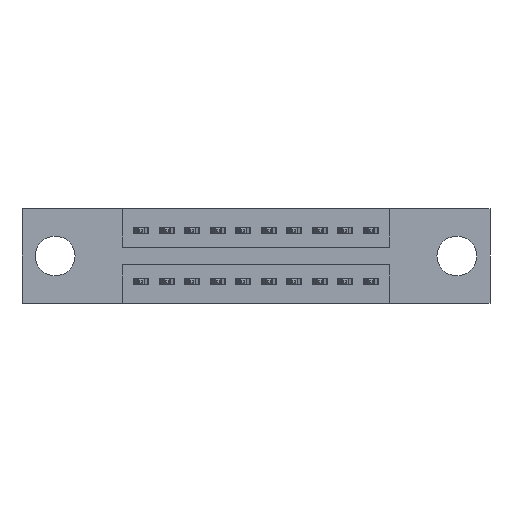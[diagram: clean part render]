
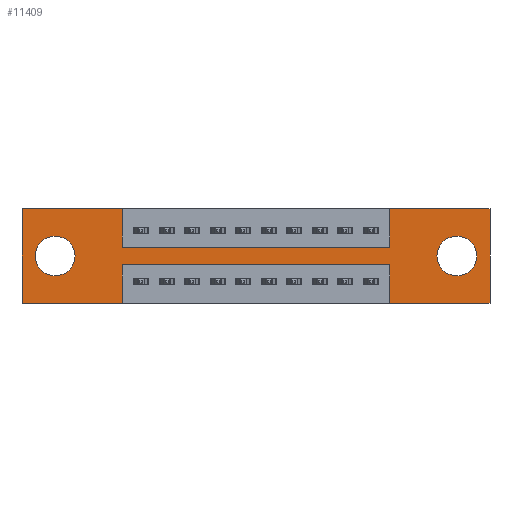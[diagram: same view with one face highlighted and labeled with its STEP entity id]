
A CAD part, front view. The second image highlights one B-rep face of the part: STEP entity #11409.
In plain terms, the highlighted planar face has unit normal (0, -1, 0).
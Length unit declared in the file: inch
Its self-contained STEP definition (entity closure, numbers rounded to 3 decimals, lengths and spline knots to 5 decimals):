
#39 = LINE ( 'NONE', #8794, #2908 ) ;
#45 = CARTESIAN_POINT ( 'NONE',  ( 0.3925, 0., -0.37 ) ) ;
#82 = CARTESIAN_POINT ( 'NONE',  ( 0., 0., 0. ) ) ;
#145 = CARTESIAN_POINT ( 'NONE',  ( 1.4425, 0., 0. ) ) ;
#156 = CARTESIAN_POINT ( 'NONE',  ( 0., 0., 0. ) ) ;
#295 = CIRCLE ( 'NONE', #908, 0.078 ) ;
#339 = DIRECTION ( 'NONE',  ( 1., 0., 0. ) ) ;
#346 = DIRECTION ( 'NONE',  ( 0., 0., 1. ) ) ;
#673 = VERTEX_POINT ( 'NONE', #9736 ) ;
#859 = ORIENTED_EDGE ( 'NONE', *, *, #5480, .T. ) ;
#908 = AXIS2_PLACEMENT_3D ( 'NONE', #1047, #8847, #7703 ) ;
#933 = LINE ( 'NONE', #156, #1925 ) ;
#968 = ORIENTED_EDGE ( 'NONE', *, *, #11265, .T. ) ;
#1047 = CARTESIAN_POINT ( 'NONE',  ( 1.705, 0., -0.185 ) ) ;
#1105 = LINE ( 'NONE', #9616, #3787 ) ;
#1170 = CARTESIAN_POINT ( 'NONE',  ( 0., 0., 0. ) ) ;
#1221 = DIRECTION ( 'NONE',  ( 0., 0., -1. ) ) ;
#1222 = ORIENTED_EDGE ( 'NONE', *, *, #12568, .T. ) ;
#1416 = VECTOR ( 'NONE', #346, 39.37008 ) ;
#1449 = LINE ( 'NONE', #5335, #8667 ) ;
#1576 = VERTEX_POINT ( 'NONE', #10463 ) ;
#1659 = PLANE ( 'NONE',  #2640 ) ;
#1796 = ORIENTED_EDGE ( 'NONE', *, *, #3796, .F. ) ;
#1900 = CARTESIAN_POINT ( 'NONE',  ( 1.4425, 0., -0.37 ) ) ;
#1903 = VERTEX_POINT ( 'NONE', #8295 ) ;
#1925 = VECTOR ( 'NONE', #5719, 39.37008 ) ;
#2301 = EDGE_CURVE ( 'NONE', #10775, #4617, #4600, .T. ) ;
#2331 = DIRECTION ( 'NONE',  ( 1., 0., 0. ) ) ;
#2640 = AXIS2_PLACEMENT_3D ( 'NONE', #3624, #9512, #3561 ) ;
#2673 = FACE_BOUND ( 'NONE', #9691, .T. ) ;
#2891 = DIRECTION ( 'NONE',  ( 0., 0., -1. ) ) ;
#2908 = VECTOR ( 'NONE', #8858, 39.37008 ) ;
#2923 = CARTESIAN_POINT ( 'NONE',  ( 0.13, 0., -0.263 ) ) ;
#3191 = EDGE_LOOP ( 'NONE', ( #4828, #6863, #5349, #1796, #12527, #7733, #8621, #10648, #10060, #8005, #12180, #5104 ) ) ;
#3241 = ORIENTED_EDGE ( 'NONE', *, *, #4675, .T. ) ;
#3254 = VERTEX_POINT ( 'NONE', #12557 ) ;
#3561 = DIRECTION ( 'NONE',  ( 0., 0., -1. ) ) ;
#3624 = CARTESIAN_POINT ( 'NONE',  ( 0., 0., -0.37 ) ) ;
#3642 = CARTESIAN_POINT ( 'NONE',  ( 0.3925, 0., -0.22 ) ) ;
#3662 = CIRCLE ( 'NONE', #6130, 0.078 ) ;
#3787 = VECTOR ( 'NONE', #11760, 39.37008 ) ;
#3796 = EDGE_CURVE ( 'NONE', #10252, #10162, #39, .T. ) ;
#3860 = CARTESIAN_POINT ( 'NONE',  ( 1.835, 0., -0.37 ) ) ;
#3870 = CARTESIAN_POINT ( 'NONE',  ( 0.3925, 0., -0.22 ) ) ;
#3967 = CARTESIAN_POINT ( 'NONE',  ( 1.835, 0., 0. ) ) ;
#4052 = DIRECTION ( 'NONE',  ( 0., 0., -1. ) ) ;
#4404 = EDGE_LOOP ( 'NONE', ( #1222, #3241 ) ) ;
#4547 = CIRCLE ( 'NONE', #5791, 0.078 ) ;
#4600 = LINE ( 'NONE', #3642, #11248 ) ;
#4617 = VERTEX_POINT ( 'NONE', #3870 ) ;
#4675 = EDGE_CURVE ( 'NONE', #9756, #10533, #4547, .T. ) ;
#4795 = EDGE_CURVE ( 'NONE', #10442, #5657, #1449, .T. ) ;
#4828 = ORIENTED_EDGE ( 'NONE', *, *, #8681, .F. ) ;
#5051 = LINE ( 'NONE', #145, #7648 ) ;
#5060 = EDGE_CURVE ( 'NONE', #1576, #10442, #933, .T. ) ;
#5104 = ORIENTED_EDGE ( 'NONE', *, *, #10304, .F. ) ;
#5241 = DIRECTION ( 'NONE',  ( 0., 0., 1. ) ) ;
#5259 = CARTESIAN_POINT ( 'NONE',  ( 0., 0., -0.37 ) ) ;
#5335 = CARTESIAN_POINT ( 'NONE',  ( 0., 0., 0. ) ) ;
#5349 = ORIENTED_EDGE ( 'NONE', *, *, #12106, .F. ) ;
#5400 = EDGE_CURVE ( 'NONE', #5657, #5859, #9602, .T. ) ;
#5480 = EDGE_CURVE ( 'NONE', #1903, #3254, #295, .T. ) ;
#5517 = VERTEX_POINT ( 'NONE', #3967 ) ;
#5569 = EDGE_CURVE ( 'NONE', #673, #5517, #11823, .T. ) ;
#5643 = EDGE_CURVE ( 'NONE', #11299, #673, #5051, .T. ) ;
#5657 = VERTEX_POINT ( 'NONE', #8964 ) ;
#5719 = DIRECTION ( 'NONE',  ( 0., 0., 1. ) ) ;
#5761 = CARTESIAN_POINT ( 'NONE',  ( 0.3925, 0., -0.15 ) ) ;
#5791 = AXIS2_PLACEMENT_3D ( 'NONE', #11146, #7072, #11018 ) ;
#5849 = LINE ( 'NONE', #9740, #1416 ) ;
#5859 = VERTEX_POINT ( 'NONE', #5761 ) ;
#5907 = VECTOR ( 'NONE', #9162, 39.37008 ) ;
#6130 = AXIS2_PLACEMENT_3D ( 'NONE', #11050, #10088, #1221 ) ;
#6332 = CARTESIAN_POINT ( 'NONE',  ( 0.13, 0., -0.185 ) ) ;
#6863 = ORIENTED_EDGE ( 'NONE', *, *, #2301, .F. ) ;
#6937 = AXIS2_PLACEMENT_3D ( 'NONE', #6332, #12198, #9024 ) ;
#7072 = DIRECTION ( 'NONE',  ( 0., 1., 0. ) ) ;
#7569 = DIRECTION ( 'NONE',  ( -1., 0., 0. ) ) ;
#7609 = EDGE_CURVE ( 'NONE', #5517, #10252, #1105, .T. ) ;
#7648 = VECTOR ( 'NONE', #5241, 39.37008 ) ;
#7703 = DIRECTION ( 'NONE',  ( 0., 0., -1. ) ) ;
#7733 = ORIENTED_EDGE ( 'NONE', *, *, #5569, .F. ) ;
#7760 = VECTOR ( 'NONE', #11075, 39.37008 ) ;
#8005 = ORIENTED_EDGE ( 'NONE', *, *, #4795, .F. ) ;
#8155 = LINE ( 'NONE', #5259, #5907 ) ;
#8295 = CARTESIAN_POINT ( 'NONE',  ( 1.705, 0., -0.107 ) ) ;
#8500 = FACE_OUTER_BOUND ( 'NONE', #3191, .T. ) ;
#8621 = ORIENTED_EDGE ( 'NONE', *, *, #5643, .F. ) ;
#8667 = VECTOR ( 'NONE', #2331, 39.37008 ) ;
#8681 = EDGE_CURVE ( 'NONE', #4617, #10199, #11852, .T. ) ;
#8794 = CARTESIAN_POINT ( 'NONE',  ( 0., 0., -0.37 ) ) ;
#8847 = DIRECTION ( 'NONE',  ( 0., 1., 0. ) ) ;
#8858 = DIRECTION ( 'NONE',  ( -1., 0., 0. ) ) ;
#8964 = CARTESIAN_POINT ( 'NONE',  ( 0.3925, 0., 0. ) ) ;
#9024 = DIRECTION ( 'NONE',  ( 0., 0., 1. ) ) ;
#9162 = DIRECTION ( 'NONE',  ( -1., 0., 0. ) ) ;
#9512 = DIRECTION ( 'NONE',  ( 0., -1., 0. ) ) ;
#9602 = LINE ( 'NONE', #10746, #12117 ) ;
#9616 = CARTESIAN_POINT ( 'NONE',  ( 1.835, 0., 0. ) ) ;
#9691 = EDGE_LOOP ( 'NONE', ( #859, #968 ) ) ;
#9736 = CARTESIAN_POINT ( 'NONE',  ( 1.4425, 0., 0. ) ) ;
#9740 = CARTESIAN_POINT ( 'NONE',  ( 1.4425, 0., -0.37 ) ) ;
#9756 = VERTEX_POINT ( 'NONE', #2923 ) ;
#9918 = CARTESIAN_POINT ( 'NONE',  ( 1.4425, 0., -0.22 ) ) ;
#9930 = LINE ( 'NONE', #10887, #7760 ) ;
#10060 = ORIENTED_EDGE ( 'NONE', *, *, #5400, .F. ) ;
#10074 = VECTOR ( 'NONE', #339, 39.37008 ) ;
#10088 = DIRECTION ( 'NONE',  ( 0., 1., 0. ) ) ;
#10162 = VERTEX_POINT ( 'NONE', #1900 ) ;
#10199 = VERTEX_POINT ( 'NONE', #45 ) ;
#10252 = VERTEX_POINT ( 'NONE', #3860 ) ;
#10283 = FACE_BOUND ( 'NONE', #4404, .T. ) ;
#10304 = EDGE_CURVE ( 'NONE', #10199, #1576, #8155, .T. ) ;
#10319 = EDGE_CURVE ( 'NONE', #5859, #11299, #9930, .T. ) ;
#10442 = VERTEX_POINT ( 'NONE', #82 ) ;
#10463 = CARTESIAN_POINT ( 'NONE',  ( 0., 0., -0.37 ) ) ;
#10533 = VERTEX_POINT ( 'NONE', #10684 ) ;
#10648 = ORIENTED_EDGE ( 'NONE', *, *, #10319, .F. ) ;
#10684 = CARTESIAN_POINT ( 'NONE',  ( 0.13, 0., -0.107 ) ) ;
#10746 = CARTESIAN_POINT ( 'NONE',  ( 0.3925, 0., 0. ) ) ;
#10755 = VECTOR ( 'NONE', #4052, 39.37008 ) ;
#10775 = VERTEX_POINT ( 'NONE', #9918 ) ;
#10887 = CARTESIAN_POINT ( 'NONE',  ( 0.3925, 0., -0.15 ) ) ;
#11018 = DIRECTION ( 'NONE',  ( 0., 0., 1. ) ) ;
#11050 = CARTESIAN_POINT ( 'NONE',  ( 1.705, 0., -0.185 ) ) ;
#11075 = DIRECTION ( 'NONE',  ( 1., 0., 0. ) ) ;
#11146 = CARTESIAN_POINT ( 'NONE',  ( 0.13, 0., -0.185 ) ) ;
#11248 = VECTOR ( 'NONE', #7569, 39.37008 ) ;
#11265 = EDGE_CURVE ( 'NONE', #3254, #1903, #3662, .T. ) ;
#11299 = VERTEX_POINT ( 'NONE', #11937 ) ;
#11409 = ADVANCED_FACE ( 'NONE', ( #2673, #10283, #8500 ), #1659, .T. ) ;
#11760 = DIRECTION ( 'NONE',  ( 0., 0., -1. ) ) ;
#11823 = LINE ( 'NONE', #1170, #10074 ) ;
#11852 = LINE ( 'NONE', #12112, #10755 ) ;
#11937 = CARTESIAN_POINT ( 'NONE',  ( 1.4425, 0., -0.15 ) ) ;
#12106 = EDGE_CURVE ( 'NONE', #10162, #10775, #5849, .T. ) ;
#12112 = CARTESIAN_POINT ( 'NONE',  ( 0.3925, 0., -0.37 ) ) ;
#12117 = VECTOR ( 'NONE', #2891, 39.37008 ) ;
#12180 = ORIENTED_EDGE ( 'NONE', *, *, #5060, .F. ) ;
#12198 = DIRECTION ( 'NONE',  ( 0., 1., 0. ) ) ;
#12424 = CIRCLE ( 'NONE', #6937, 0.078 ) ;
#12527 = ORIENTED_EDGE ( 'NONE', *, *, #7609, .F. ) ;
#12557 = CARTESIAN_POINT ( 'NONE',  ( 1.705, 0., -0.263 ) ) ;
#12568 = EDGE_CURVE ( 'NONE', #10533, #9756, #12424, .T. ) ;
